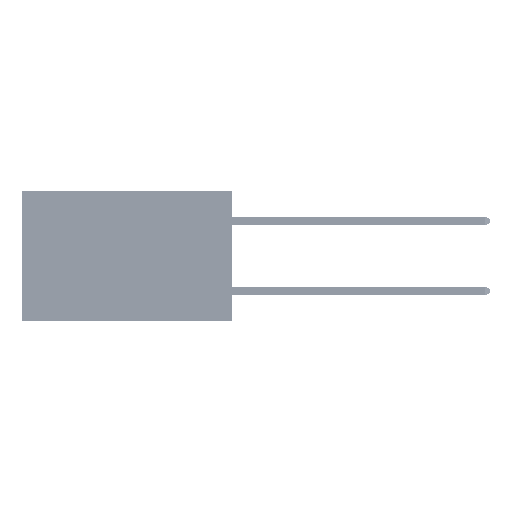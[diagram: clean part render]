
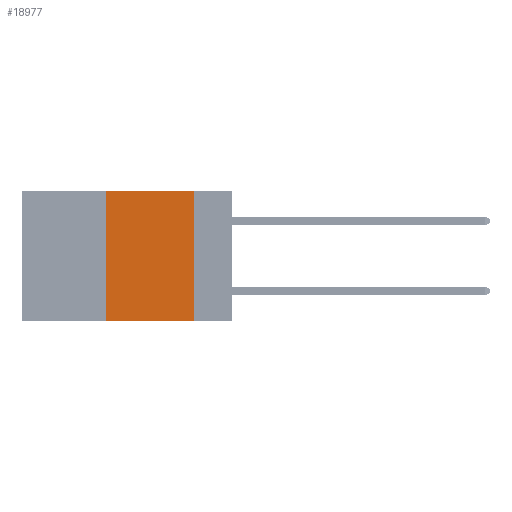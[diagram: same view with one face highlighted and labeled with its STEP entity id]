
A CAD part, left-side view. The second image highlights one B-rep face of the part: STEP entity #18977.
In plain terms, the highlighted planar face has unit normal (-1, 0, 0).
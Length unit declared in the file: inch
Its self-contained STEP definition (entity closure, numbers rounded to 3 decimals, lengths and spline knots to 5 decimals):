
#166 = EDGE_CURVE ( 'NONE', #15536, #2522, #13867, .T. ) ;
#2522 = VERTEX_POINT ( 'NONE', #45265 ) ;
#3128 = AXIS2_PLACEMENT_3D ( 'NONE', #23014, #30554, #17922 ) ;
#3537 = DIRECTION ( 'NONE',  ( 0., -1., 0. ) ) ;
#5846 = ORIENTED_EDGE ( 'NONE', *, *, #36840, .T. ) ;
#6446 = VECTOR ( 'NONE', #38634, 39.37008 ) ;
#11933 = ORIENTED_EDGE ( 'NONE', *, *, #48076, .F. ) ;
#12260 = LINE ( 'NONE', #16829, #12901 ) ;
#12437 = VERTEX_POINT ( 'NONE', #14429 ) ;
#12901 = VECTOR ( 'NONE', #41014, 39.37008 ) ;
#13867 = LINE ( 'NONE', #30293, #17826 ) ;
#14429 = CARTESIAN_POINT ( 'NONE',  ( 0., 0.36, -0.37 ) ) ;
#15536 = VERTEX_POINT ( 'NONE', #51008 ) ;
#15887 = LINE ( 'NONE', #40626, #22220 ) ;
#16829 = CARTESIAN_POINT ( 'NONE',  ( 0., 0.6, 0. ) ) ;
#17354 = ORIENTED_EDGE ( 'NONE', *, *, #40995, .F. ) ;
#17826 = VECTOR ( 'NONE', #46654, 39.37008 ) ;
#17922 = DIRECTION ( 'NONE',  ( 0., 0., -1. ) ) ;
#18977 = ADVANCED_FACE ( 'NONE', ( #42621 ), #31077, .F. ) ;
#20373 = VERTEX_POINT ( 'NONE', #23074 ) ;
#21545 = EDGE_LOOP ( 'NONE', ( #45466, #17354, #11933, #5846 ) ) ;
#22220 = VECTOR ( 'NONE', #3537, 39.37008 ) ;
#22285 = CARTESIAN_POINT ( 'NONE',  ( 0., 0.36, 0. ) ) ;
#23014 = CARTESIAN_POINT ( 'NONE',  ( 0., 0.6, 0. ) ) ;
#23074 = CARTESIAN_POINT ( 'NONE',  ( 0., 0.36, 0. ) ) ;
#30293 = CARTESIAN_POINT ( 'NONE',  ( 0., 0.11, 0. ) ) ;
#30554 = DIRECTION ( 'NONE',  ( 1., 0., 0. ) ) ;
#31077 = PLANE ( 'NONE',  #3128 ) ;
#36840 = EDGE_CURVE ( 'NONE', #12437, #2522, #15887, .T. ) ;
#38634 = DIRECTION ( 'NONE',  ( 0., 0., 1. ) ) ;
#40626 = CARTESIAN_POINT ( 'NONE',  ( 0., 0.6, -0.37 ) ) ;
#40995 = EDGE_CURVE ( 'NONE', #20373, #15536, #12260, .T. ) ;
#41014 = DIRECTION ( 'NONE',  ( 0., -1., 0. ) ) ;
#42621 = FACE_OUTER_BOUND ( 'NONE', #21545, .T. ) ;
#43458 = LINE ( 'NONE', #22285, #6446 ) ;
#45265 = CARTESIAN_POINT ( 'NONE',  ( 0., 0.11, -0.37 ) ) ;
#45466 = ORIENTED_EDGE ( 'NONE', *, *, #166, .F. ) ;
#46654 = DIRECTION ( 'NONE',  ( 0., 0., -1. ) ) ;
#48076 = EDGE_CURVE ( 'NONE', #12437, #20373, #43458, .T. ) ;
#51008 = CARTESIAN_POINT ( 'NONE',  ( 0., 0.11, 0. ) ) ;
